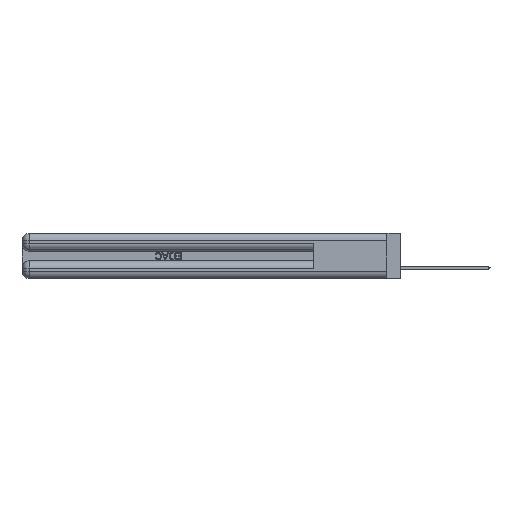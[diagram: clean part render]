
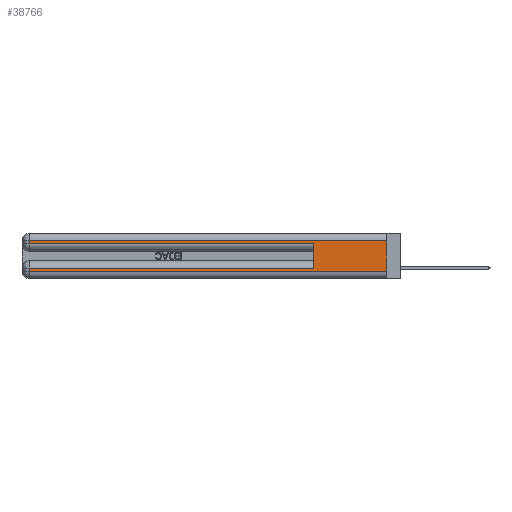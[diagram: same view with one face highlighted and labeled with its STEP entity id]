
A CAD part, left-side view. The second image highlights one B-rep face of the part: STEP entity #38766.
In plain terms, the highlighted planar face has unit normal (-1, 0, 0).
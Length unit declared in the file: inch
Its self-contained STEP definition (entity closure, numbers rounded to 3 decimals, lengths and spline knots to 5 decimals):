
#978 = VERTEX_POINT ( 'NONE', #15168 ) ;
#1222 = CARTESIAN_POINT ( 'NONE',  ( 0., 2.94, 0.06 ) ) ;
#1819 = CARTESIAN_POINT ( 'NONE',  ( 0., 0.6, 0.145 ) ) ;
#1946 = FACE_OUTER_BOUND ( 'NONE', #9242, .T. ) ;
#2016 = DIRECTION ( 'NONE',  ( 0., -1., 0. ) ) ;
#2092 = CARTESIAN_POINT ( 'NONE',  ( 0., 0., 0.31 ) ) ;
#2192 = CARTESIAN_POINT ( 'NONE',  ( 0., 0., 0.285 ) ) ;
#3694 = EDGE_CURVE ( 'NONE', #45296, #18100, #28110, .T. ) ;
#4619 = VECTOR ( 'NONE', #32171, 39.37008 ) ;
#4681 = CARTESIAN_POINT ( 'NONE',  ( 0., 0., 0.31 ) ) ;
#5184 = PLANE ( 'NONE',  #20004 ) ;
#7031 = EDGE_CURVE ( 'NONE', #21042, #37777, #47518, .T. ) ;
#9242 = EDGE_LOOP ( 'NONE', ( #48974, #47591, #39680, #11843, #31858, #25326, #42221, #41360 ) ) ;
#10203 = CARTESIAN_POINT ( 'NONE',  ( 0., 0., 0.06 ) ) ;
#10391 = VECTOR ( 'NONE', #24902, 39.37008 ) ;
#10461 = EDGE_CURVE ( 'NONE', #45296, #33869, #39194, .T. ) ;
#10465 = EDGE_CURVE ( 'NONE', #44836, #37777, #33252, .T. ) ;
#11469 = VECTOR ( 'NONE', #36937, 39.37008 ) ;
#11843 = ORIENTED_EDGE ( 'NONE', *, *, #7031, .T. ) ;
#12556 = DIRECTION ( 'NONE',  ( 0., 1., 0. ) ) ;
#15168 = CARTESIAN_POINT ( 'NONE',  ( 0., 2.94, 0.085 ) ) ;
#16177 = DIRECTION ( 'NONE',  ( 0., 1., 0. ) ) ;
#17992 = CARTESIAN_POINT ( 'NONE',  ( 0., 0., 0.085 ) ) ;
#18100 = VERTEX_POINT ( 'NONE', #10203 ) ;
#19157 = CARTESIAN_POINT ( 'NONE',  ( 0., 0.6, 0.285 ) ) ;
#20004 = AXIS2_PLACEMENT_3D ( 'NONE', #20542, #40014, #28689 ) ;
#20542 = CARTESIAN_POINT ( 'NONE',  ( 0., 0., 0.37 ) ) ;
#21042 = VERTEX_POINT ( 'NONE', #34018 ) ;
#22867 = LINE ( 'NONE', #29591, #11469 ) ;
#24232 = CARTESIAN_POINT ( 'NONE',  ( 0., 2.94, 0.37 ) ) ;
#24902 = DIRECTION ( 'NONE',  ( 0., 0., -1. ) ) ;
#25326 = ORIENTED_EDGE ( 'NONE', *, *, #39098, .T. ) ;
#25414 = DIRECTION ( 'NONE',  ( 0., 0., -1. ) ) ;
#25534 = VECTOR ( 'NONE', #16177, 39.37008 ) ;
#25860 = LINE ( 'NONE', #17992, #38338 ) ;
#28110 = LINE ( 'NONE', #40251, #38273 ) ;
#28689 = DIRECTION ( 'NONE',  ( 0., 0., -1. ) ) ;
#29591 = CARTESIAN_POINT ( 'NONE',  ( 0., 0., 0.06 ) ) ;
#31858 = ORIENTED_EDGE ( 'NONE', *, *, #10465, .F. ) ;
#32171 = DIRECTION ( 'NONE',  ( 0., 0., 1. ) ) ;
#32520 = EDGE_CURVE ( 'NONE', #34894, #18100, #22867, .T. ) ;
#32767 = DIRECTION ( 'NONE',  ( 0., 0., -1. ) ) ;
#32880 = CARTESIAN_POINT ( 'NONE',  ( 0., 2.94, 0.37 ) ) ;
#33252 = LINE ( 'NONE', #1819, #4619 ) ;
#33869 = VERTEX_POINT ( 'NONE', #44234 ) ;
#34018 = CARTESIAN_POINT ( 'NONE',  ( 0., 2.94, 0.285 ) ) ;
#34349 = CARTESIAN_POINT ( 'NONE',  ( 0., 0.6, 0.085 ) ) ;
#34894 = VERTEX_POINT ( 'NONE', #1222 ) ;
#36937 = DIRECTION ( 'NONE',  ( 0., -1., 0. ) ) ;
#37777 = VERTEX_POINT ( 'NONE', #19157 ) ;
#38273 = VECTOR ( 'NONE', #32767, 39.37008 ) ;
#38338 = VECTOR ( 'NONE', #12556, 39.37008 ) ;
#38766 = ADVANCED_FACE ( 'NONE', ( #1946 ), #5184, .F. ) ;
#39098 = EDGE_CURVE ( 'NONE', #44836, #978, #25860, .T. ) ;
#39194 = LINE ( 'NONE', #4681, #25534 ) ;
#39680 = ORIENTED_EDGE ( 'NONE', *, *, #42788, .T. ) ;
#40014 = DIRECTION ( 'NONE',  ( 1., 0., 0. ) ) ;
#40251 = CARTESIAN_POINT ( 'NONE',  ( 0., 0., 0.37 ) ) ;
#41360 = ORIENTED_EDGE ( 'NONE', *, *, #32520, .T. ) ;
#42221 = ORIENTED_EDGE ( 'NONE', *, *, #45713, .T. ) ;
#42788 = EDGE_CURVE ( 'NONE', #33869, #21042, #48858, .T. ) ;
#44234 = CARTESIAN_POINT ( 'NONE',  ( 0., 2.94, 0.31 ) ) ;
#44836 = VERTEX_POINT ( 'NONE', #34349 ) ;
#45296 = VERTEX_POINT ( 'NONE', #2092 ) ;
#45578 = LINE ( 'NONE', #24232, #10391 ) ;
#45713 = EDGE_CURVE ( 'NONE', #978, #34894, #45578, .T. ) ;
#47518 = LINE ( 'NONE', #2192, #49308 ) ;
#47591 = ORIENTED_EDGE ( 'NONE', *, *, #10461, .T. ) ;
#47636 = VECTOR ( 'NONE', #25414, 39.37008 ) ;
#48858 = LINE ( 'NONE', #32880, #47636 ) ;
#48974 = ORIENTED_EDGE ( 'NONE', *, *, #3694, .F. ) ;
#49308 = VECTOR ( 'NONE', #2016, 39.37008 ) ;
